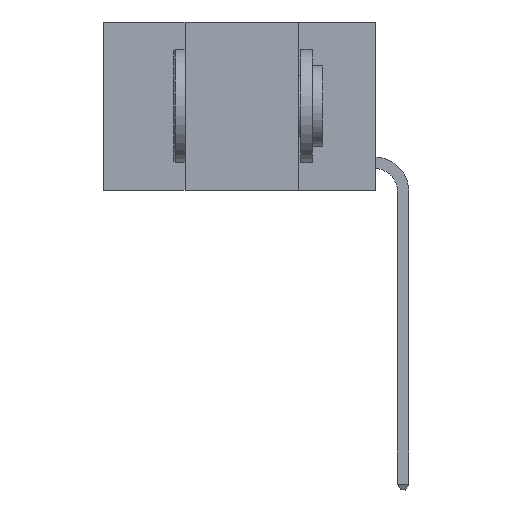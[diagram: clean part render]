
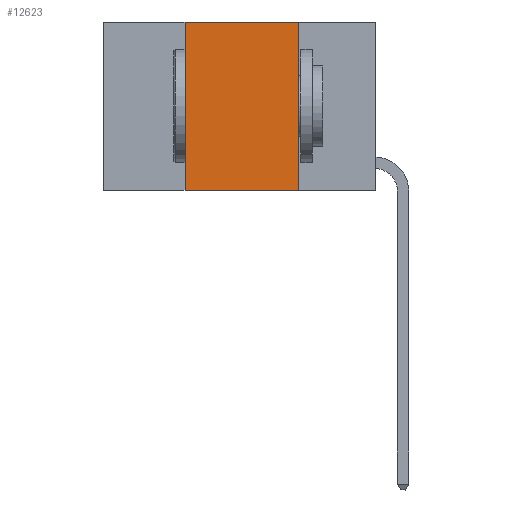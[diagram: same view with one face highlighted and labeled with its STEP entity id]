
A CAD part, left-side view. The second image highlights one B-rep face of the part: STEP entity #12623.
In plain terms, the highlighted planar face has unit normal (-1, 0, 0).
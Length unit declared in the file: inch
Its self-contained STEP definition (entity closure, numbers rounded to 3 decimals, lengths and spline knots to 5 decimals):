
#224 = CARTESIAN_POINT ( 'NONE',  ( 0., 0.6, -0.37 ) ) ;
#288 = LINE ( 'NONE', #6615, #13332 ) ;
#711 = PLANE ( 'NONE',  #9659 ) ;
#758 = EDGE_CURVE ( 'NONE', #5627, #6596, #11430, .T. ) ;
#1519 = DIRECTION ( 'NONE',  ( 0., -1., 0. ) ) ;
#1739 = EDGE_CURVE ( 'NONE', #5309, #10894, #288, .T. ) ;
#2140 = LINE ( 'NONE', #224, #8534 ) ;
#2941 = VECTOR ( 'NONE', #14180, 39.37008 ) ;
#4660 = DIRECTION ( 'NONE',  ( 0., 0., -1. ) ) ;
#5055 = ORIENTED_EDGE ( 'NONE', *, *, #758, .F. ) ;
#5309 = VERTEX_POINT ( 'NONE', #13589 ) ;
#5456 = ORIENTED_EDGE ( 'NONE', *, *, #6743, .T. ) ;
#5627 = VERTEX_POINT ( 'NONE', #10523 ) ;
#6135 = CARTESIAN_POINT ( 'NONE',  ( 0., 0.6, 0. ) ) ;
#6596 = VERTEX_POINT ( 'NONE', #13808 ) ;
#6615 = CARTESIAN_POINT ( 'NONE',  ( 0., 0.17, 0. ) ) ;
#6743 = EDGE_CURVE ( 'NONE', #5627, #10894, #2140, .T. ) ;
#8534 = VECTOR ( 'NONE', #1519, 39.37008 ) ;
#9177 = LINE ( 'NONE', #6135, #15695 ) ;
#9659 = AXIS2_PLACEMENT_3D ( 'NONE', #10913, #12118, #4660 ) ;
#10523 = CARTESIAN_POINT ( 'NONE',  ( 0., 0.42, -0.37 ) ) ;
#10894 = VERTEX_POINT ( 'NONE', #16066 ) ;
#10913 = CARTESIAN_POINT ( 'NONE',  ( 0., 0.6, 0. ) ) ;
#11313 = ORIENTED_EDGE ( 'NONE', *, *, #1739, .F. ) ;
#11430 = LINE ( 'NONE', #13347, #2941 ) ;
#12118 = DIRECTION ( 'NONE',  ( 1., 0., 0. ) ) ;
#12623 = ADVANCED_FACE ( 'NONE', ( #14675 ), #711, .F. ) ;
#13332 = VECTOR ( 'NONE', #15724, 39.37008 ) ;
#13347 = CARTESIAN_POINT ( 'NONE',  ( 0., 0.42, 0. ) ) ;
#13372 = EDGE_CURVE ( 'NONE', #6596, #5309, #9177, .T. ) ;
#13589 = CARTESIAN_POINT ( 'NONE',  ( 0., 0.17, 0. ) ) ;
#13808 = CARTESIAN_POINT ( 'NONE',  ( 0., 0.42, 0. ) ) ;
#14102 = EDGE_LOOP ( 'NONE', ( #11313, #14554, #5055, #5456 ) ) ;
#14180 = DIRECTION ( 'NONE',  ( 0., 0., 1. ) ) ;
#14554 = ORIENTED_EDGE ( 'NONE', *, *, #13372, .F. ) ;
#14675 = FACE_OUTER_BOUND ( 'NONE', #14102, .T. ) ;
#14769 = DIRECTION ( 'NONE',  ( 0., -1., 0. ) ) ;
#15695 = VECTOR ( 'NONE', #14769, 39.37008 ) ;
#15724 = DIRECTION ( 'NONE',  ( 0., 0., -1. ) ) ;
#16066 = CARTESIAN_POINT ( 'NONE',  ( 0., 0.17, -0.37 ) ) ;
